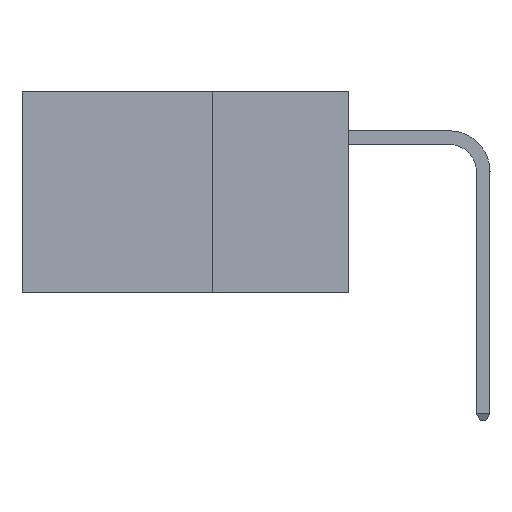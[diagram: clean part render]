
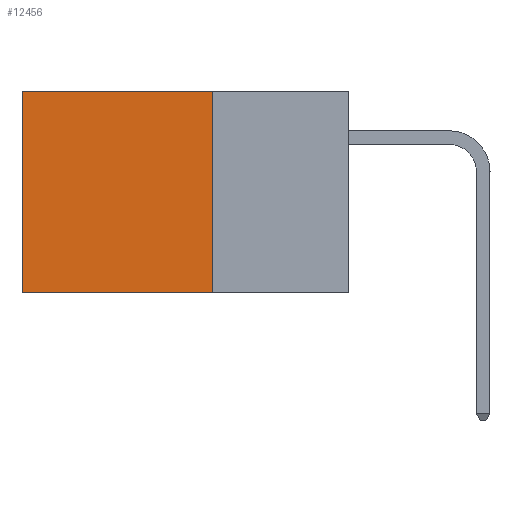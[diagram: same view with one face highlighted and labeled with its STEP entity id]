
A CAD part, left-side view. The second image highlights one B-rep face of the part: STEP entity #12456.
In plain terms, the highlighted planar face has unit normal (-1, 0, 0).
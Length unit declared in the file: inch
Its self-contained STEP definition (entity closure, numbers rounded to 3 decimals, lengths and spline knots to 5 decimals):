
#2415 = VERTEX_POINT ( 'NONE', #26379 ) ;
#3723 = CARTESIAN_POINT ( 'NONE',  ( 0.2875, 0.25, -0.37 ) ) ;
#4039 = VERTEX_POINT ( 'NONE', #36083 ) ;
#4158 = LINE ( 'NONE', #17928, #40787 ) ;
#5814 = VECTOR ( 'NONE', #18292, 39.37008 ) ;
#6120 = CARTESIAN_POINT ( 'NONE',  ( 0.2875, 0.25, -0.37 ) ) ;
#6413 = EDGE_LOOP ( 'NONE', ( #16359, #12881, #32554, #19599 ) ) ;
#7891 = VECTOR ( 'NONE', #34322, 39.37008 ) ;
#9107 = DIRECTION ( 'NONE',  ( 1., 0., 0. ) ) ;
#12400 = AXIS2_PLACEMENT_3D ( 'NONE', #36780, #9107, #31050 ) ;
#12456 = ADVANCED_FACE ( 'NONE', ( #16373 ), #33575, .F. ) ;
#12881 = ORIENTED_EDGE ( 'NONE', *, *, #13394, .F. ) ;
#13394 = EDGE_CURVE ( 'NONE', #31690, #22434, #13826, .T. ) ;
#13826 = LINE ( 'NONE', #6120, #7891 ) ;
#14157 = EDGE_CURVE ( 'NONE', #4039, #22434, #25075, .T. ) ;
#15545 = DIRECTION ( 'NONE',  ( 0., 1., 0. ) ) ;
#16188 = EDGE_CURVE ( 'NONE', #2415, #4039, #4158, .T. ) ;
#16359 = ORIENTED_EDGE ( 'NONE', *, *, #14157, .T. ) ;
#16373 = FACE_OUTER_BOUND ( 'NONE', #6413, .T. ) ;
#16906 = VECTOR ( 'NONE', #30805, 39.37008 ) ;
#17928 = CARTESIAN_POINT ( 'NONE',  ( 0.2875, 0.25, 0. ) ) ;
#17937 = LINE ( 'NONE', #21403, #16906 ) ;
#18292 = DIRECTION ( 'NONE',  ( 0., 0., -1. ) ) ;
#19599 = ORIENTED_EDGE ( 'NONE', *, *, #16188, .T. ) ;
#21403 = CARTESIAN_POINT ( 'NONE',  ( 0.2875, 0.25, 0. ) ) ;
#22434 = VERTEX_POINT ( 'NONE', #40490 ) ;
#24243 = EDGE_CURVE ( 'NONE', #2415, #31690, #17937, .T. ) ;
#25075 = LINE ( 'NONE', #28028, #5814 ) ;
#26379 = CARTESIAN_POINT ( 'NONE',  ( 0.2875, 0.25, 0. ) ) ;
#28028 = CARTESIAN_POINT ( 'NONE',  ( 0.2875, 0.6, 0. ) ) ;
#30805 = DIRECTION ( 'NONE',  ( 0., 0., -1. ) ) ;
#31050 = DIRECTION ( 'NONE',  ( 0., 0., -1. ) ) ;
#31690 = VERTEX_POINT ( 'NONE', #3723 ) ;
#32554 = ORIENTED_EDGE ( 'NONE', *, *, #24243, .F. ) ;
#33575 = PLANE ( 'NONE',  #12400 ) ;
#34322 = DIRECTION ( 'NONE',  ( 0., 1., 0. ) ) ;
#36083 = CARTESIAN_POINT ( 'NONE',  ( 0.2875, 0.6, 0. ) ) ;
#36780 = CARTESIAN_POINT ( 'NONE',  ( 0.2875, 0.25, 0. ) ) ;
#40490 = CARTESIAN_POINT ( 'NONE',  ( 0.2875, 0.6, -0.37 ) ) ;
#40787 = VECTOR ( 'NONE', #15545, 39.37008 ) ;
